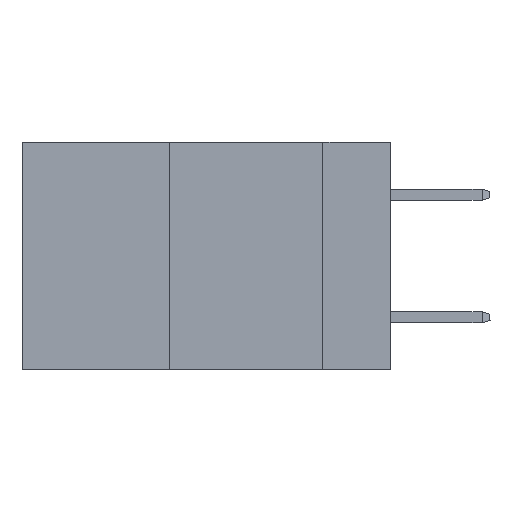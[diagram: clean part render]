
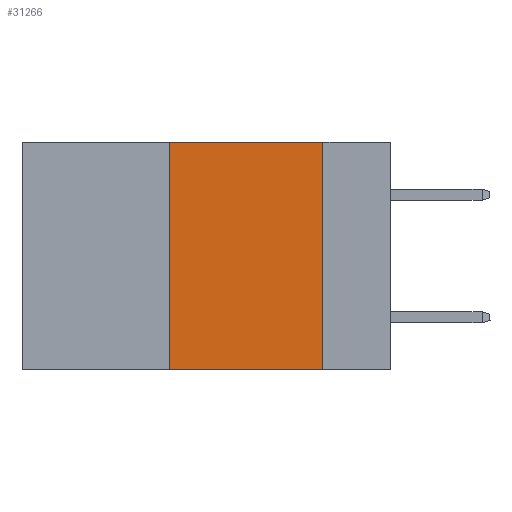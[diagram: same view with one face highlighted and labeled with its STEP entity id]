
A CAD part, left-side view. The second image highlights one B-rep face of the part: STEP entity #31266.
In plain terms, the highlighted planar face has unit normal (-1, 0, 0).
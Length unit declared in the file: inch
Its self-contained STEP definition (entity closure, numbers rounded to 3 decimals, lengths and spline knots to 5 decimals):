
#268 = EDGE_CURVE ( 'NONE', #26002, #29327, #7076, .T. ) ;
#276 = DIRECTION ( 'NONE',  ( 1., 0., 0. ) ) ;
#966 = CARTESIAN_POINT ( 'NONE',  ( 0., 0.11, -0.37 ) ) ;
#3293 = CARTESIAN_POINT ( 'NONE',  ( 0., 0.36, 0. ) ) ;
#3320 = CARTESIAN_POINT ( 'NONE',  ( 0., 0.6, 0. ) ) ;
#3500 = VECTOR ( 'NONE', #28916, 39.37008 ) ;
#4403 = EDGE_LOOP ( 'NONE', ( #20705, #28915, #22838, #9925 ) ) ;
#4815 = CARTESIAN_POINT ( 'NONE',  ( 0., 0.11, 0. ) ) ;
#5789 = LINE ( 'NONE', #3293, #3500 ) ;
#6107 = CARTESIAN_POINT ( 'NONE',  ( 0., 0.11, 0. ) ) ;
#7076 = LINE ( 'NONE', #34025, #15146 ) ;
#8737 = CARTESIAN_POINT ( 'NONE',  ( 0., 0.6, -0.37 ) ) ;
#9925 = ORIENTED_EDGE ( 'NONE', *, *, #23384, .T. ) ;
#11484 = DIRECTION ( 'NONE',  ( 0., -1., 0. ) ) ;
#11652 = LINE ( 'NONE', #4815, #20606 ) ;
#14005 = VECTOR ( 'NONE', #11484, 39.37008 ) ;
#15146 = VECTOR ( 'NONE', #19826, 39.37008 ) ;
#15998 = FACE_OUTER_BOUND ( 'NONE', #4403, .T. ) ;
#16933 = VERTEX_POINT ( 'NONE', #966 ) ;
#19826 = DIRECTION ( 'NONE',  ( 0., -1., 0. ) ) ;
#20571 = PLANE ( 'NONE',  #36338 ) ;
#20606 = VECTOR ( 'NONE', #33826, 39.37008 ) ;
#20705 = ORIENTED_EDGE ( 'NONE', *, *, #27242, .F. ) ;
#21195 = DIRECTION ( 'NONE',  ( 0., 0., -1. ) ) ;
#22838 = ORIENTED_EDGE ( 'NONE', *, *, #35716, .F. ) ;
#23384 = EDGE_CURVE ( 'NONE', #36821, #16933, #31885, .T. ) ;
#26002 = VERTEX_POINT ( 'NONE', #34893 ) ;
#27242 = EDGE_CURVE ( 'NONE', #29327, #16933, #11652, .T. ) ;
#28915 = ORIENTED_EDGE ( 'NONE', *, *, #268, .F. ) ;
#28916 = DIRECTION ( 'NONE',  ( 0., 0., 1. ) ) ;
#28946 = CARTESIAN_POINT ( 'NONE',  ( 0., 0.36, -0.37 ) ) ;
#29327 = VERTEX_POINT ( 'NONE', #6107 ) ;
#31266 = ADVANCED_FACE ( 'NONE', ( #15998 ), #20571, .F. ) ;
#31885 = LINE ( 'NONE', #8737, #14005 ) ;
#33826 = DIRECTION ( 'NONE',  ( 0., 0., -1. ) ) ;
#34025 = CARTESIAN_POINT ( 'NONE',  ( 0., 0.6, 0. ) ) ;
#34893 = CARTESIAN_POINT ( 'NONE',  ( 0., 0.36, 0. ) ) ;
#35716 = EDGE_CURVE ( 'NONE', #36821, #26002, #5789, .T. ) ;
#36338 = AXIS2_PLACEMENT_3D ( 'NONE', #3320, #276, #21195 ) ;
#36821 = VERTEX_POINT ( 'NONE', #28946 ) ;
